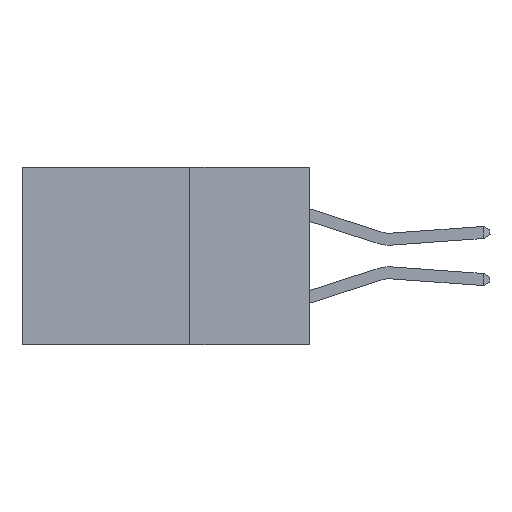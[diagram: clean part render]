
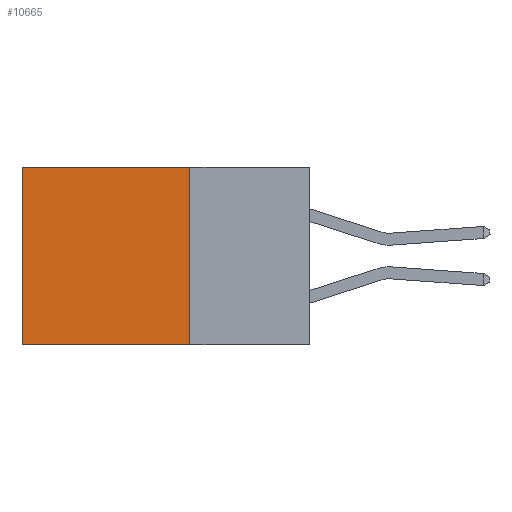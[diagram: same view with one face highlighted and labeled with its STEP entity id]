
A CAD part, left-side view. The second image highlights one B-rep face of the part: STEP entity #10665.
In plain terms, the highlighted planar face has unit normal (-1, 0, 0).
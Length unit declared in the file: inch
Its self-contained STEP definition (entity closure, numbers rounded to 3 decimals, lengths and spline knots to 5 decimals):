
#903 = LINE ( 'NONE', #21648, #4794 ) ;
#1668 = DIRECTION ( 'NONE',  ( 0., 1., 0. ) ) ;
#2306 = VERTEX_POINT ( 'NONE', #13737 ) ;
#2728 = CARTESIAN_POINT ( 'NONE',  ( 0.2615, 0.25, -0.37 ) ) ;
#3881 = DIRECTION ( 'NONE',  ( 0., 0., -1. ) ) ;
#4319 = EDGE_CURVE ( 'NONE', #5716, #17493, #8354, .T. ) ;
#4794 = VECTOR ( 'NONE', #3881, 39.37008 ) ;
#5361 = CARTESIAN_POINT ( 'NONE',  ( 0.2615, 0.25, -0.37 ) ) ;
#5716 = VERTEX_POINT ( 'NONE', #11643 ) ;
#5746 = ORIENTED_EDGE ( 'NONE', *, *, #11617, .T. ) ;
#6516 = DIRECTION ( 'NONE',  ( 0., 0., -1. ) ) ;
#8060 = VECTOR ( 'NONE', #11527, 39.37008 ) ;
#8071 = ORIENTED_EDGE ( 'NONE', *, *, #4319, .F. ) ;
#8130 = CARTESIAN_POINT ( 'NONE',  ( 0.2615, 0.25, -0.37 ) ) ;
#8354 = LINE ( 'NONE', #8130, #14833 ) ;
#9540 = DIRECTION ( 'NONE',  ( 0., 0., -1. ) ) ;
#10665 = ADVANCED_FACE ( 'NONE', ( #14662 ), #21588, .F. ) ;
#11166 = CARTESIAN_POINT ( 'NONE',  ( 0.2615, 0.6, -0.37 ) ) ;
#11432 = VECTOR ( 'NONE', #1668, 39.37008 ) ;
#11527 = DIRECTION ( 'NONE',  ( 0., 1., 0. ) ) ;
#11617 = EDGE_CURVE ( 'NONE', #5716, #2306, #19327, .T. ) ;
#11643 = CARTESIAN_POINT ( 'NONE',  ( 0.2615, 0.25, 0. ) ) ;
#12592 = VERTEX_POINT ( 'NONE', #11166 ) ;
#12950 = CARTESIAN_POINT ( 'NONE',  ( 0.2615, 0.25, -0.37 ) ) ;
#13681 = ORIENTED_EDGE ( 'NONE', *, *, #21115, .T. ) ;
#13737 = CARTESIAN_POINT ( 'NONE',  ( 0.2615, 0.6, 0. ) ) ;
#13746 = AXIS2_PLACEMENT_3D ( 'NONE', #12950, #18188, #9540 ) ;
#14662 = FACE_OUTER_BOUND ( 'NONE', #20975, .T. ) ;
#14833 = VECTOR ( 'NONE', #6516, 39.37008 ) ;
#15819 = CARTESIAN_POINT ( 'NONE',  ( 0.2615, 0.25, 0. ) ) ;
#17493 = VERTEX_POINT ( 'NONE', #5361 ) ;
#18188 = DIRECTION ( 'NONE',  ( 1., 0., 0. ) ) ;
#18361 = LINE ( 'NONE', #2728, #8060 ) ;
#19236 = EDGE_CURVE ( 'NONE', #17493, #12592, #18361, .T. ) ;
#19327 = LINE ( 'NONE', #15819, #11432 ) ;
#20381 = ORIENTED_EDGE ( 'NONE', *, *, #19236, .F. ) ;
#20975 = EDGE_LOOP ( 'NONE', ( #13681, #20381, #8071, #5746 ) ) ;
#21115 = EDGE_CURVE ( 'NONE', #2306, #12592, #903, .T. ) ;
#21588 = PLANE ( 'NONE',  #13746 ) ;
#21648 = CARTESIAN_POINT ( 'NONE',  ( 0.2615, 0.6, -0.37 ) ) ;
